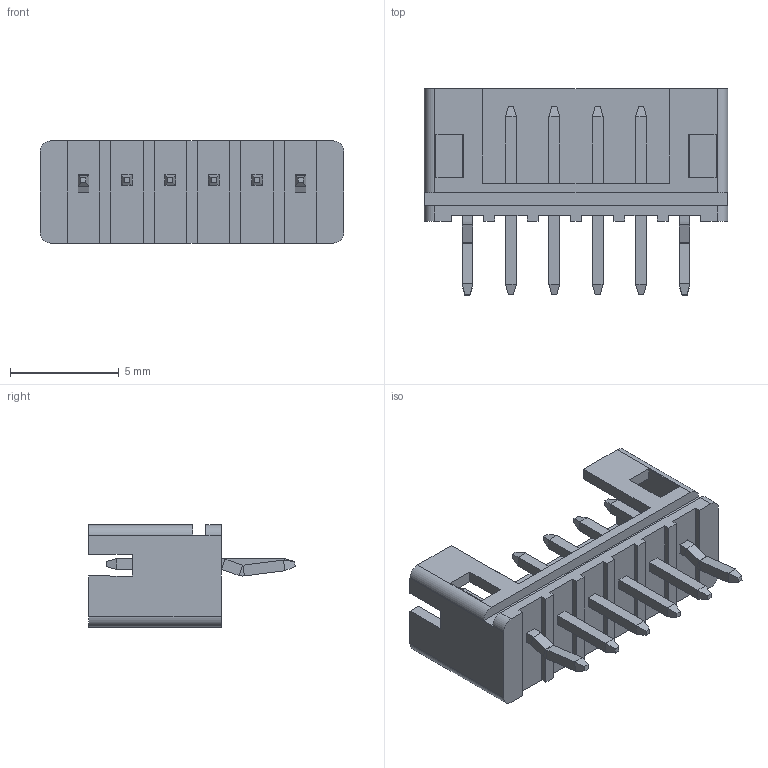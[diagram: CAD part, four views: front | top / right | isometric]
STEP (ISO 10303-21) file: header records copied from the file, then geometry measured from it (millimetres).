
FILE_DESCRIPTION (( 'STEP AP203' ), '1' );
FILE_NAME ('140-506-415-001.STEP', '2020-03-31T19:21:50', ( '' ), ( '' ), 'SwSTEP 2.0', 'SolidWorks 2016', '' );
FILE_SCHEMA (( 'CONFIG_CONTROL_DESIGN' ));
Length unit declared in the file: millimetre
Products named in the file (4): 140-506-415-001; V Housing_506; V Contact_Kink; V Contact_Str
Assembly tree (7 placements, depth 2):
  140-506-415-001
    V Housing_506
    V Contact_Kink  x2
    V Contact_Str  x4
Bounding box: 14 x 9.51 x 4.7 mm (x, y, z)
Volume: 157 mm3; surface area: 576.5 mm2
Topology: 7 solids, 7 shells, 202 faces, 498 edges, 308 vertices
Faces by surface type: plane 184, cylinder 16, bspline 2
Entity records: 4595 total; most frequent: CARTESIAN_POINT 751, ORIENTED_EDGE 702, DIRECTION 655, EDGE_CURVE 351, LINE 327, VECTOR 327, VERTEX_POINT 224, AXIS2_PLACEMENT_3D 164
